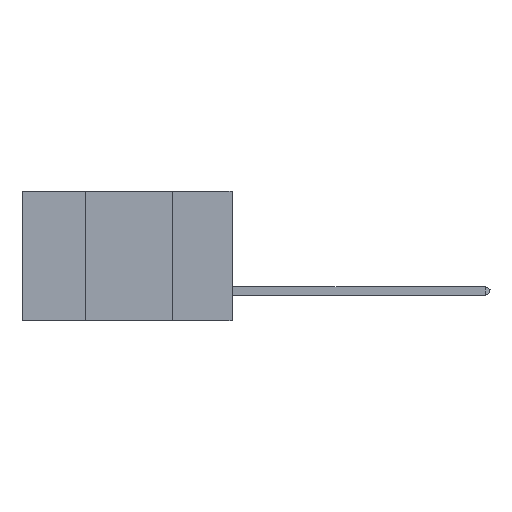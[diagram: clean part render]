
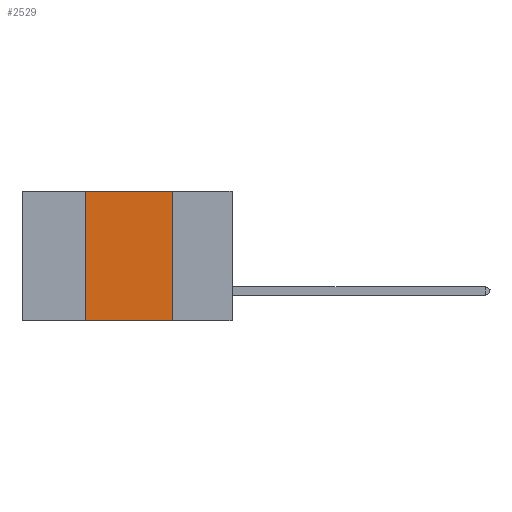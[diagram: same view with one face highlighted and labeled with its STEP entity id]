
A CAD part, left-side view. The second image highlights one B-rep face of the part: STEP entity #2529.
In plain terms, the highlighted planar face has unit normal (-1, 0, 0).
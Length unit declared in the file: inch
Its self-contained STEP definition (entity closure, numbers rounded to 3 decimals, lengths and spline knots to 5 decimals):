
#388 = VERTEX_POINT ( 'NONE', #5080 ) ;
#979 = VECTOR ( 'NONE', #5604, 39.37008 ) ;
#1150 = FACE_OUTER_BOUND ( 'NONE', #8285, .T. ) ;
#1183 = VERTEX_POINT ( 'NONE', #4765 ) ;
#1438 = CARTESIAN_POINT ( 'NONE',  ( 0., 0.42, 0. ) ) ;
#1442 = DIRECTION ( 'NONE',  ( 1., 0., 0. ) ) ;
#2040 = LINE ( 'NONE', #5066, #10442 ) ;
#2529 = ADVANCED_FACE ( 'NONE', ( #1150 ), #6937, .F. ) ;
#2725 = EDGE_CURVE ( 'NONE', #4669, #5227, #4698, .T. ) ;
#2847 = AXIS2_PLACEMENT_3D ( 'NONE', #9387, #1442, #8772 ) ;
#3417 = VECTOR ( 'NONE', #8363, 39.37008 ) ;
#3537 = EDGE_CURVE ( 'NONE', #5227, #1183, #4305, .T. ) ;
#4099 = CARTESIAN_POINT ( 'NONE',  ( 0., 0.6, 0. ) ) ;
#4305 = LINE ( 'NONE', #7551, #3417 ) ;
#4474 = ORIENTED_EDGE ( 'NONE', *, *, #9486, .T. ) ;
#4669 = VERTEX_POINT ( 'NONE', #1438 ) ;
#4698 = LINE ( 'NONE', #4099, #9439 ) ;
#4765 = CARTESIAN_POINT ( 'NONE',  ( 0., 0.17, -0.37 ) ) ;
#5066 = CARTESIAN_POINT ( 'NONE',  ( 0., 0.42, 0. ) ) ;
#5080 = CARTESIAN_POINT ( 'NONE',  ( 0., 0.42, -0.37 ) ) ;
#5227 = VERTEX_POINT ( 'NONE', #5963 ) ;
#5604 = DIRECTION ( 'NONE',  ( 0., -1., 0. ) ) ;
#5963 = CARTESIAN_POINT ( 'NONE',  ( 0., 0.17, 0. ) ) ;
#6349 = CARTESIAN_POINT ( 'NONE',  ( 0., 0.6, -0.37 ) ) ;
#6454 = DIRECTION ( 'NONE',  ( 0., -1., 0. ) ) ;
#6689 = DIRECTION ( 'NONE',  ( 0., 0., 1. ) ) ;
#6937 = PLANE ( 'NONE',  #2847 ) ;
#7551 = CARTESIAN_POINT ( 'NONE',  ( 0., 0.17, 0. ) ) ;
#8262 = ORIENTED_EDGE ( 'NONE', *, *, #8863, .F. ) ;
#8285 = EDGE_LOOP ( 'NONE', ( #9318, #9503, #8262, #4474 ) ) ;
#8363 = DIRECTION ( 'NONE',  ( 0., 0., -1. ) ) ;
#8507 = LINE ( 'NONE', #6349, #979 ) ;
#8772 = DIRECTION ( 'NONE',  ( 0., 0., -1. ) ) ;
#8863 = EDGE_CURVE ( 'NONE', #388, #4669, #2040, .T. ) ;
#9318 = ORIENTED_EDGE ( 'NONE', *, *, #3537, .F. ) ;
#9387 = CARTESIAN_POINT ( 'NONE',  ( 0., 0.6, 0. ) ) ;
#9439 = VECTOR ( 'NONE', #6454, 39.37008 ) ;
#9486 = EDGE_CURVE ( 'NONE', #388, #1183, #8507, .T. ) ;
#9503 = ORIENTED_EDGE ( 'NONE', *, *, #2725, .F. ) ;
#10442 = VECTOR ( 'NONE', #6689, 39.37008 ) ;
